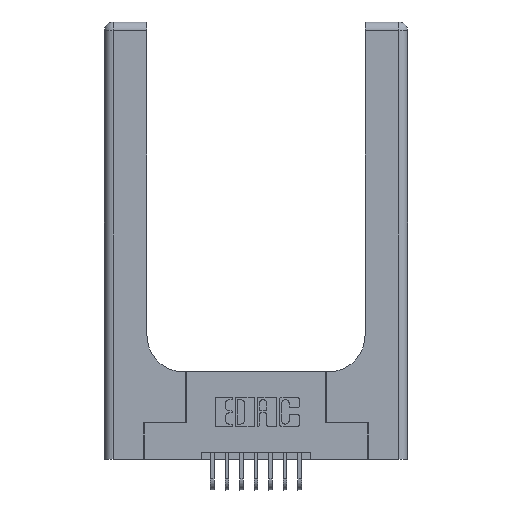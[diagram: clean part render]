
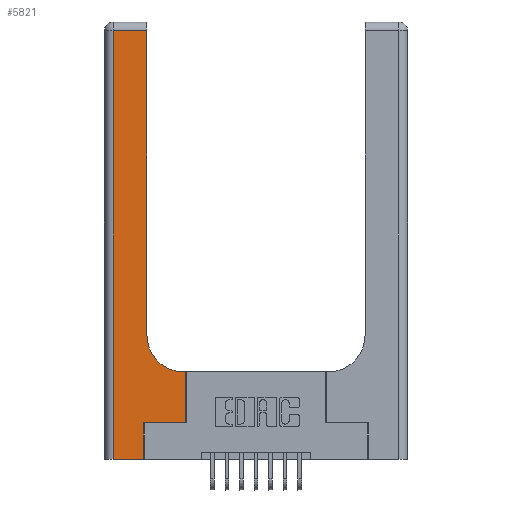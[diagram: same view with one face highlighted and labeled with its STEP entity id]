
A CAD part, top view. The second image highlights one B-rep face of the part: STEP entity #5821.
In plain terms, the highlighted planar face has unit normal (0, 0, 1).
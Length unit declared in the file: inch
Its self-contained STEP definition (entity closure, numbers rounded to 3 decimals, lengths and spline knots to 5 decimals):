
#45 = DIRECTION ( 'NONE',  ( 0., 0., -1. ) ) ;
#266 = CARTESIAN_POINT ( 'NONE',  ( 0.5585, 0.25, 0.37 ) ) ;
#286 = EDGE_CURVE ( 'NONE', #5249, #14105, #14442, .T. ) ;
#314 = ORIENTED_EDGE ( 'NONE', *, *, #14108, .T. ) ;
#532 = PLANE ( 'NONE',  #15716 ) ;
#743 = EDGE_LOOP ( 'NONE', ( #6364, #14408, #5715, #5455, #7903, #6897, #14584, #14546, #314 ) ) ;
#763 = CARTESIAN_POINT ( 'NONE',  ( 0.06, 3., 0.37 ) ) ;
#1157 = CARTESIAN_POINT ( 'NONE',  ( 0.5585, 0.6, 0.37 ) ) ;
#1458 = CARTESIAN_POINT ( 'NONE',  ( 0.269, 0.25, 0.37 ) ) ;
#1745 = VECTOR ( 'NONE', #8370, 39.37008 ) ;
#1956 = DIRECTION ( 'NONE',  ( -1., 0., 0. ) ) ;
#2418 = EDGE_CURVE ( 'NONE', #3296, #11676, #15599, .T. ) ;
#2928 = VECTOR ( 'NONE', #9962, 39.37008 ) ;
#3196 = AXIS2_PLACEMENT_3D ( 'NONE', #3874, #45, #9207 ) ;
#3296 = VERTEX_POINT ( 'NONE', #16042 ) ;
#3777 = VECTOR ( 'NONE', #1956, 39.37008 ) ;
#3874 = CARTESIAN_POINT ( 'NONE',  ( 0.5415, 0.85, 0.37 ) ) ;
#3924 = EDGE_CURVE ( 'NONE', #15078, #5249, #5836, .T. ) ;
#4543 = CARTESIAN_POINT ( 'NONE',  ( 0.06, 2.94, 0.37 ) ) ;
#4673 = VECTOR ( 'NONE', #15358, 39.37008 ) ;
#4763 = CARTESIAN_POINT ( 'NONE',  ( 0., 3., 0.37 ) ) ;
#5018 = CARTESIAN_POINT ( 'NONE',  ( 0., 2.94, 0.37 ) ) ;
#5249 = VERTEX_POINT ( 'NONE', #15105 ) ;
#5406 = CARTESIAN_POINT ( 'NONE',  ( 0.5415, 0.6, 0.37 ) ) ;
#5455 = ORIENTED_EDGE ( 'NONE', *, *, #3924, .T. ) ;
#5715 = ORIENTED_EDGE ( 'NONE', *, *, #17048, .T. ) ;
#5775 = DIRECTION ( 'NONE',  ( 0., 1., 0. ) ) ;
#5821 = ADVANCED_FACE ( 'NONE', ( #12368 ), #532, .F. ) ;
#5836 = LINE ( 'NONE', #8322, #1745 ) ;
#6000 = CARTESIAN_POINT ( 'NONE',  ( 0.269, 0.25, 0.37 ) ) ;
#6364 = ORIENTED_EDGE ( 'NONE', *, *, #2418, .T. ) ;
#6733 = CARTESIAN_POINT ( 'NONE',  ( 0.269, 0., 0.37 ) ) ;
#6897 = ORIENTED_EDGE ( 'NONE', *, *, #7155, .T. ) ;
#7155 = EDGE_CURVE ( 'NONE', #14105, #11043, #15236, .T. ) ;
#7903 = ORIENTED_EDGE ( 'NONE', *, *, #286, .T. ) ;
#8229 = VERTEX_POINT ( 'NONE', #5406 ) ;
#8322 = CARTESIAN_POINT ( 'NONE',  ( 0., 0., 0.37 ) ) ;
#8370 = DIRECTION ( 'NONE',  ( 1., 0., 0. ) ) ;
#8613 = VECTOR ( 'NONE', #11351, 39.37008 ) ;
#9107 = DIRECTION ( 'NONE',  ( 0., 1., 0. ) ) ;
#9207 = DIRECTION ( 'NONE',  ( 1., 0., 0. ) ) ;
#9734 = EDGE_CURVE ( 'NONE', #11676, #15876, #10250, .T. ) ;
#9822 = CARTESIAN_POINT ( 'NONE',  ( 0.2915, 0.6, 0.37 ) ) ;
#9866 = CARTESIAN_POINT ( 'NONE',  ( 0.5585, 0.25, 0.37 ) ) ;
#9962 = DIRECTION ( 'NONE',  ( 0., -1., 0. ) ) ;
#10129 = LINE ( 'NONE', #763, #2928 ) ;
#10250 = LINE ( 'NONE', #5018, #4673 ) ;
#11043 = VERTEX_POINT ( 'NONE', #266 ) ;
#11351 = DIRECTION ( 'NONE',  ( 1., 0., 0. ) ) ;
#11498 = CARTESIAN_POINT ( 'NONE',  ( 0.2915, 3., 0.37 ) ) ;
#11562 = LINE ( 'NONE', #9866, #16157 ) ;
#11676 = VERTEX_POINT ( 'NONE', #14855 ) ;
#11799 = LINE ( 'NONE', #9822, #3777 ) ;
#11888 = CARTESIAN_POINT ( 'NONE',  ( 0.06, 0., 0.37 ) ) ;
#11964 = DIRECTION ( 'NONE',  ( 0., 1., 0. ) ) ;
#12058 = VECTOR ( 'NONE', #9107, 39.37008 ) ;
#12368 = FACE_OUTER_BOUND ( 'NONE', #743, .T. ) ;
#12684 = VERTEX_POINT ( 'NONE', #1157 ) ;
#12788 = VECTOR ( 'NONE', #11964, 39.37008 ) ;
#13979 = DIRECTION ( 'NONE',  ( -1., 0., 0. ) ) ;
#14105 = VERTEX_POINT ( 'NONE', #1458 ) ;
#14108 = EDGE_CURVE ( 'NONE', #8229, #3296, #15676, .T. ) ;
#14408 = ORIENTED_EDGE ( 'NONE', *, *, #9734, .T. ) ;
#14442 = LINE ( 'NONE', #6733, #12788 ) ;
#14546 = ORIENTED_EDGE ( 'NONE', *, *, #16026, .T. ) ;
#14584 = ORIENTED_EDGE ( 'NONE', *, *, #16520, .T. ) ;
#14855 = CARTESIAN_POINT ( 'NONE',  ( 0.2915, 2.94, 0.37 ) ) ;
#15078 = VERTEX_POINT ( 'NONE', #11888 ) ;
#15105 = CARTESIAN_POINT ( 'NONE',  ( 0.269, 0., 0.37 ) ) ;
#15236 = LINE ( 'NONE', #6000, #8613 ) ;
#15358 = DIRECTION ( 'NONE',  ( -1., 0., 0. ) ) ;
#15391 = DIRECTION ( 'NONE',  ( 0., 0., -1. ) ) ;
#15599 = LINE ( 'NONE', #11498, #12058 ) ;
#15676 = CIRCLE ( 'NONE', #3196, 0.25 ) ;
#15716 = AXIS2_PLACEMENT_3D ( 'NONE', #4763, #15391, #13979 ) ;
#15876 = VERTEX_POINT ( 'NONE', #4543 ) ;
#16026 = EDGE_CURVE ( 'NONE', #12684, #8229, #11799, .T. ) ;
#16042 = CARTESIAN_POINT ( 'NONE',  ( 0.2915, 0.85, 0.37 ) ) ;
#16157 = VECTOR ( 'NONE', #5775, 39.37008 ) ;
#16520 = EDGE_CURVE ( 'NONE', #11043, #12684, #11562, .T. ) ;
#17048 = EDGE_CURVE ( 'NONE', #15876, #15078, #10129, .T. ) ;
